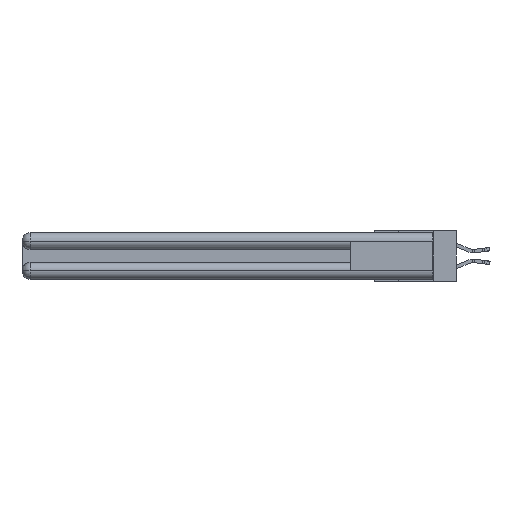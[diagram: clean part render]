
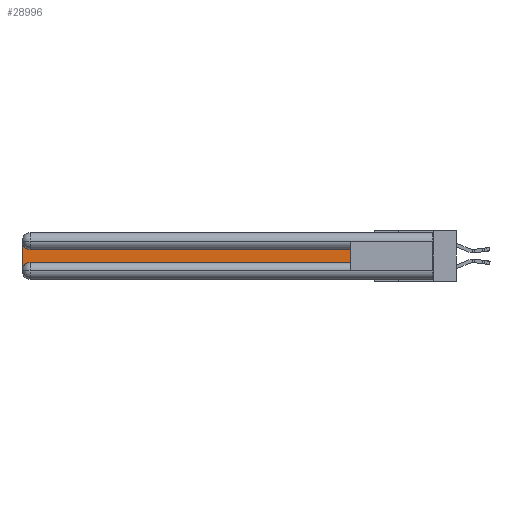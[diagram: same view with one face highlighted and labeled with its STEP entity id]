
A CAD part, left-side view. The second image highlights one B-rep face of the part: STEP entity #28996.
In plain terms, the highlighted planar face has unit normal (-1, 0, 0).
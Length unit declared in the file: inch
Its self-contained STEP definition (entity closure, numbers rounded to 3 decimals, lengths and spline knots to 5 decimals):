
#465 = VERTEX_POINT ( 'NONE', #18096 ) ;
#1921 = DIRECTION ( 'NONE',  ( 0., 1., 0. ) ) ;
#3464 = EDGE_CURVE ( 'NONE', #27525, #20597, #25014, .T. ) ;
#3810 = CARTESIAN_POINT ( 'NONE',  ( 0.075, 3., -0.2175 ) ) ;
#4194 = DIRECTION ( 'NONE',  ( 1., 0., 0. ) ) ;
#4408 = DIRECTION ( 'NONE',  ( 0., 0., -1. ) ) ;
#4603 = CIRCLE ( 'NONE', #19846, 0.06 ) ;
#4923 = EDGE_CURVE ( 'NONE', #20597, #465, #4603, .T. ) ;
#5259 = CIRCLE ( 'NONE', #18274, 0.06 ) ;
#5831 = ORIENTED_EDGE ( 'NONE', *, *, #27815, .T. ) ;
#5967 = EDGE_CURVE ( 'NONE', #465, #18700, #12205, .T. ) ;
#7630 = VECTOR ( 'NONE', #24611, 39.37008 ) ;
#7738 = CARTESIAN_POINT ( 'NONE',  ( 0.075, 0.6, -0.2175 ) ) ;
#8023 = LINE ( 'NONE', #8361, #7630 ) ;
#8361 = CARTESIAN_POINT ( 'NONE',  ( 0.075, 0.6, -0.2175 ) ) ;
#8930 = CARTESIAN_POINT ( 'NONE',  ( 0.075, 2.94, -0.1225 ) ) ;
#9537 = CARTESIAN_POINT ( 'NONE',  ( 0.075, 0.6, -0.1225 ) ) ;
#9810 = CARTESIAN_POINT ( 'NONE',  ( 0.075, 0.6, -0.2175 ) ) ;
#10994 = CARTESIAN_POINT ( 'NONE',  ( 0.075, 3., -0.2775 ) ) ;
#11826 = EDGE_CURVE ( 'NONE', #18700, #30543, #5259, .T. ) ;
#12205 = LINE ( 'NONE', #3810, #24065 ) ;
#12909 = ORIENTED_EDGE ( 'NONE', *, *, #5967, .T. ) ;
#13328 = CARTESIAN_POINT ( 'NONE',  ( 0.075, 2.94, -0.0625 ) ) ;
#15595 = LINE ( 'NONE', #7738, #31404 ) ;
#15850 = CARTESIAN_POINT ( 'NONE',  ( 0.075, 0.6, -0.1225 ) ) ;
#15933 = FACE_OUTER_BOUND ( 'NONE', #22733, .T. ) ;
#16561 = VECTOR ( 'NONE', #1921, 39.37008 ) ;
#16567 = ORIENTED_EDGE ( 'NONE', *, *, #3464, .T. ) ;
#17154 = PLANE ( 'NONE',  #27251 ) ;
#17345 = ORIENTED_EDGE ( 'NONE', *, *, #4923, .T. ) ;
#17450 = ORIENTED_EDGE ( 'NONE', *, *, #28428, .T. ) ;
#18096 = CARTESIAN_POINT ( 'NONE',  ( 0.075, 3., -0.0625 ) ) ;
#18151 = DIRECTION ( 'NONE',  ( 1., 0., 0. ) ) ;
#18274 = AXIS2_PLACEMENT_3D ( 'NONE', #28566, #4194, #4408 ) ;
#18700 = VERTEX_POINT ( 'NONE', #10994 ) ;
#19846 = AXIS2_PLACEMENT_3D ( 'NONE', #13328, #18151, #30217 ) ;
#20281 = VERTEX_POINT ( 'NONE', #9810 ) ;
#20597 = VERTEX_POINT ( 'NONE', #8930 ) ;
#20765 = DIRECTION ( 'NONE',  ( 0., -1., 0. ) ) ;
#22130 = CARTESIAN_POINT ( 'NONE',  ( 0.075, 2.94, -0.2175 ) ) ;
#22733 = EDGE_LOOP ( 'NONE', ( #16567, #17345, #12909, #28270, #17450, #5831 ) ) ;
#24065 = VECTOR ( 'NONE', #28507, 39.37008 ) ;
#24611 = DIRECTION ( 'NONE',  ( 0., 0., 1. ) ) ;
#25014 = LINE ( 'NONE', #9537, #16561 ) ;
#27251 = AXIS2_PLACEMENT_3D ( 'NONE', #29655, #29549, #29441 ) ;
#27525 = VERTEX_POINT ( 'NONE', #15850 ) ;
#27815 = EDGE_CURVE ( 'NONE', #20281, #27525, #8023, .T. ) ;
#28270 = ORIENTED_EDGE ( 'NONE', *, *, #11826, .T. ) ;
#28428 = EDGE_CURVE ( 'NONE', #30543, #20281, #15595, .T. ) ;
#28507 = DIRECTION ( 'NONE',  ( 0., 0., -1. ) ) ;
#28566 = CARTESIAN_POINT ( 'NONE',  ( 0.075, 2.94, -0.2775 ) ) ;
#28996 = ADVANCED_FACE ( 'NONE', ( #15933 ), #17154, .F. ) ;
#29441 = DIRECTION ( 'NONE',  ( 0., 0., -1. ) ) ;
#29549 = DIRECTION ( 'NONE',  ( 1., 0., 0. ) ) ;
#29655 = CARTESIAN_POINT ( 'NONE',  ( 0.075, 3., -0.1225 ) ) ;
#30217 = DIRECTION ( 'NONE',  ( 0., 0., -1. ) ) ;
#30543 = VERTEX_POINT ( 'NONE', #22130 ) ;
#31404 = VECTOR ( 'NONE', #20765, 39.37008 ) ;
